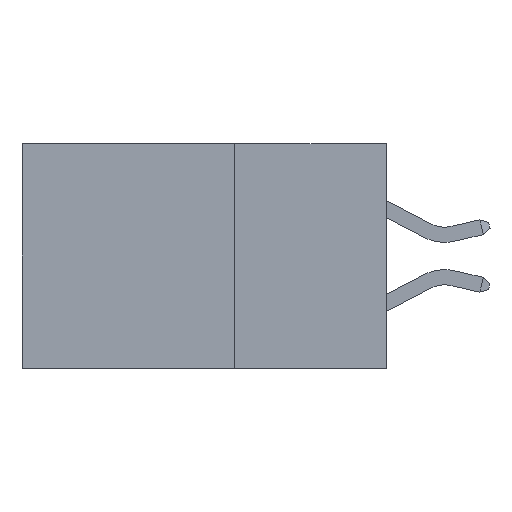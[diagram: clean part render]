
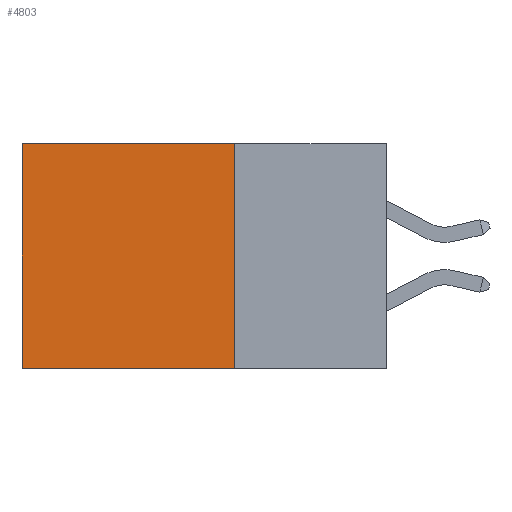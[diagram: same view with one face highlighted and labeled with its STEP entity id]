
A CAD part, left-side view. The second image highlights one B-rep face of the part: STEP entity #4803.
In plain terms, the highlighted planar face has unit normal (-1, 0, 0).
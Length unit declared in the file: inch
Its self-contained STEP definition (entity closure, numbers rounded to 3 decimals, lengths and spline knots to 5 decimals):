
#706 = DIRECTION ( 'NONE',  ( 0., 1., 0. ) ) ;
#995 = EDGE_CURVE ( 'NONE', #9302, #5853, #4813, .T. ) ;
#1363 = VECTOR ( 'NONE', #4532, 39.37008 ) ;
#2018 = LINE ( 'NONE', #9108, #5914 ) ;
#2030 = CARTESIAN_POINT ( 'NONE',  ( 0.298, 0.25, 0. ) ) ;
#2934 = VERTEX_POINT ( 'NONE', #2030 ) ;
#3262 = PLANE ( 'NONE',  #6700 ) ;
#3660 = CARTESIAN_POINT ( 'NONE',  ( 0.298, 0.25, 0. ) ) ;
#4532 = DIRECTION ( 'NONE',  ( 0., 1., 0. ) ) ;
#4803 = ADVANCED_FACE ( 'NONE', ( #10233 ), #3262, .F. ) ;
#4813 = LINE ( 'NONE', #17765, #1363 ) ;
#5853 = VERTEX_POINT ( 'NONE', #9106 ) ;
#5914 = VECTOR ( 'NONE', #6275, 39.37008 ) ;
#6198 = DIRECTION ( 'NONE',  ( 0., 0., -1. ) ) ;
#6275 = DIRECTION ( 'NONE',  ( 0., 0., -1. ) ) ;
#6700 = AXIS2_PLACEMENT_3D ( 'NONE', #13262, #14658, #6198 ) ;
#6730 = EDGE_CURVE ( 'NONE', #2934, #9302, #15455, .T. ) ;
#6800 = ORIENTED_EDGE ( 'NONE', *, *, #16734, .T. ) ;
#7098 = VERTEX_POINT ( 'NONE', #16954 ) ;
#7213 = ORIENTED_EDGE ( 'NONE', *, *, #995, .F. ) ;
#8073 = CARTESIAN_POINT ( 'NONE',  ( 0.298, 0.25, 0. ) ) ;
#8180 = ORIENTED_EDGE ( 'NONE', *, *, #12302, .T. ) ;
#9106 = CARTESIAN_POINT ( 'NONE',  ( 0.298, 0.6, -0.37 ) ) ;
#9108 = CARTESIAN_POINT ( 'NONE',  ( 0.298, 0.6, 0. ) ) ;
#9302 = VERTEX_POINT ( 'NONE', #16000 ) ;
#9330 = LINE ( 'NONE', #3660, #16823 ) ;
#10233 = FACE_OUTER_BOUND ( 'NONE', #15957, .T. ) ;
#11730 = VECTOR ( 'NONE', #17948, 39.37008 ) ;
#12302 = EDGE_CURVE ( 'NONE', #2934, #7098, #9330, .T. ) ;
#13262 = CARTESIAN_POINT ( 'NONE',  ( 0.298, 0.25, 0. ) ) ;
#13818 = ORIENTED_EDGE ( 'NONE', *, *, #6730, .F. ) ;
#14658 = DIRECTION ( 'NONE',  ( 1., 0., 0. ) ) ;
#15455 = LINE ( 'NONE', #8073, #11730 ) ;
#15957 = EDGE_LOOP ( 'NONE', ( #6800, #7213, #13818, #8180 ) ) ;
#16000 = CARTESIAN_POINT ( 'NONE',  ( 0.298, 0.25, -0.37 ) ) ;
#16734 = EDGE_CURVE ( 'NONE', #7098, #5853, #2018, .T. ) ;
#16823 = VECTOR ( 'NONE', #706, 39.37008 ) ;
#16954 = CARTESIAN_POINT ( 'NONE',  ( 0.298, 0.6, 0. ) ) ;
#17765 = CARTESIAN_POINT ( 'NONE',  ( 0.298, 0.25, -0.37 ) ) ;
#17948 = DIRECTION ( 'NONE',  ( 0., 0., -1. ) ) ;
